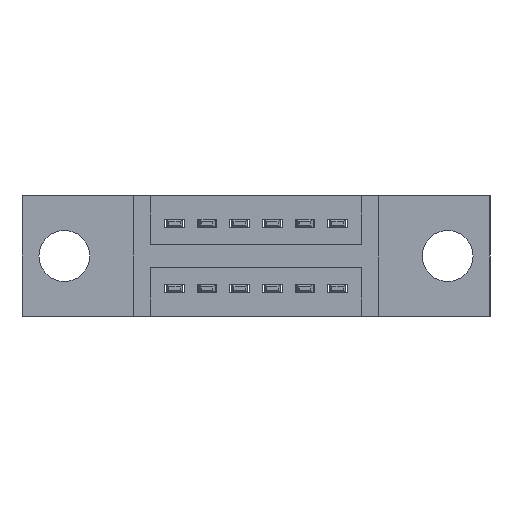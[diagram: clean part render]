
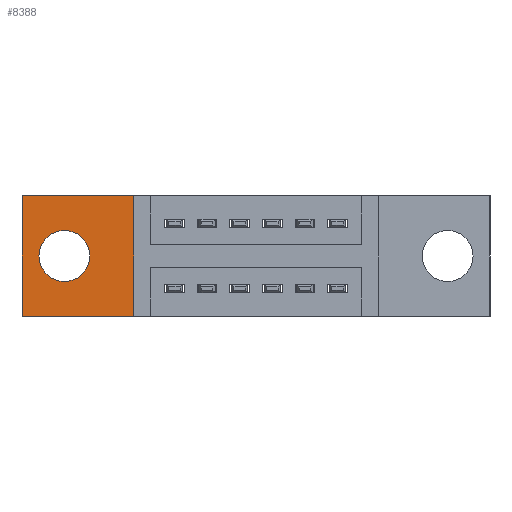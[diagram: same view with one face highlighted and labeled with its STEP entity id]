
A CAD part, front view. The second image highlights one B-rep face of the part: STEP entity #8388.
In plain terms, the highlighted planar face has unit normal (0, -1, 0).
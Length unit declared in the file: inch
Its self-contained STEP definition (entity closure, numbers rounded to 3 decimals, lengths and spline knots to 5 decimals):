
#304 = AXIS2_PLACEMENT_3D ( 'NONE', #477, #456, #7009 ) ;
#371 = AXIS2_PLACEMENT_3D ( 'NONE', #6355, #4152, #2954 ) ;
#456 = DIRECTION ( 'NONE',  ( 0., -1., 0. ) ) ;
#477 = CARTESIAN_POINT ( 'NONE',  ( 0., 0.17, -0.37 ) ) ;
#710 = VERTEX_POINT ( 'NONE', #9398 ) ;
#741 = EDGE_CURVE ( 'NONE', #1641, #5937, #3170, .T. ) ;
#893 = VECTOR ( 'NONE', #1954, 39.37008 ) ;
#1215 = CARTESIAN_POINT ( 'NONE',  ( 0.13, 0.17, -0.107 ) ) ;
#1598 = ORIENTED_EDGE ( 'NONE', *, *, #5074, .F. ) ;
#1641 = VERTEX_POINT ( 'NONE', #6620 ) ;
#1666 = CARTESIAN_POINT ( 'NONE',  ( 0., 0.17, 0. ) ) ;
#1954 = DIRECTION ( 'NONE',  ( 0., 0., -1. ) ) ;
#1985 = CARTESIAN_POINT ( 'NONE',  ( 0., 0.17, 0. ) ) ;
#2731 = PLANE ( 'NONE',  #304 ) ;
#2954 = DIRECTION ( 'NONE',  ( 0., 0., -1. ) ) ;
#3034 = CIRCLE ( 'NONE', #371, 0.078 ) ;
#3081 = ORIENTED_EDGE ( 'NONE', *, *, #9248, .F. ) ;
#3170 = LINE ( 'NONE', #1985, #893 ) ;
#3262 = AXIS2_PLACEMENT_3D ( 'NONE', #3743, #4475, #5957 ) ;
#3398 = VERTEX_POINT ( 'NONE', #1215 ) ;
#3563 = CARTESIAN_POINT ( 'NONE',  ( 0., 0.17, -0.37 ) ) ;
#3608 = VERTEX_POINT ( 'NONE', #4558 ) ;
#3743 = CARTESIAN_POINT ( 'NONE',  ( 0.13, 0.17, -0.185 ) ) ;
#3832 = DIRECTION ( 'NONE',  ( -1., 0., 0. ) ) ;
#3960 = VECTOR ( 'NONE', #3832, 39.37008 ) ;
#4073 = ORIENTED_EDGE ( 'NONE', *, *, #4602, .T. ) ;
#4152 = DIRECTION ( 'NONE',  ( 0., -1., 0. ) ) ;
#4201 = LINE ( 'NONE', #4662, #7805 ) ;
#4475 = DIRECTION ( 'NONE',  ( 0., -1., 0. ) ) ;
#4529 = ORIENTED_EDGE ( 'NONE', *, *, #741, .T. ) ;
#4558 = CARTESIAN_POINT ( 'NONE',  ( 0.13, 0.17, -0.263 ) ) ;
#4602 = EDGE_CURVE ( 'NONE', #5937, #710, #6333, .T. ) ;
#4662 = CARTESIAN_POINT ( 'NONE',  ( 0.3425, 0.17, 0. ) ) ;
#4689 = ORIENTED_EDGE ( 'NONE', *, *, #7722, .T. ) ;
#4899 = CARTESIAN_POINT ( 'NONE',  ( 0.3425, 0.17, 0. ) ) ;
#5042 = EDGE_LOOP ( 'NONE', ( #1598, #3081 ) ) ;
#5074 = EDGE_CURVE ( 'NONE', #3398, #3608, #6286, .T. ) ;
#5295 = EDGE_CURVE ( 'NONE', #8436, #1641, #9396, .T. ) ;
#5647 = EDGE_LOOP ( 'NONE', ( #4529, #4073, #4689, #7973 ) ) ;
#5930 = VECTOR ( 'NONE', #6534, 39.37008 ) ;
#5937 = VERTEX_POINT ( 'NONE', #3563 ) ;
#5957 = DIRECTION ( 'NONE',  ( 0., 0., -1. ) ) ;
#6045 = CARTESIAN_POINT ( 'NONE',  ( 0., 0.17, -0.37 ) ) ;
#6090 = DIRECTION ( 'NONE',  ( 0., 0., 1. ) ) ;
#6286 = CIRCLE ( 'NONE', #3262, 0.078 ) ;
#6333 = LINE ( 'NONE', #6045, #5930 ) ;
#6355 = CARTESIAN_POINT ( 'NONE',  ( 0.13, 0.17, -0.185 ) ) ;
#6378 = FACE_BOUND ( 'NONE', #5042, .T. ) ;
#6534 = DIRECTION ( 'NONE',  ( 1., 0., 0. ) ) ;
#6620 = CARTESIAN_POINT ( 'NONE',  ( 0., 0.17, 0. ) ) ;
#7009 = DIRECTION ( 'NONE',  ( 0., 0., -1. ) ) ;
#7550 = FACE_OUTER_BOUND ( 'NONE', #5647, .T. ) ;
#7722 = EDGE_CURVE ( 'NONE', #710, #8436, #4201, .T. ) ;
#7805 = VECTOR ( 'NONE', #6090, 39.37008 ) ;
#7973 = ORIENTED_EDGE ( 'NONE', *, *, #5295, .T. ) ;
#8388 = ADVANCED_FACE ( 'NONE', ( #6378, #7550 ), #2731, .T. ) ;
#8436 = VERTEX_POINT ( 'NONE', #4899 ) ;
#9248 = EDGE_CURVE ( 'NONE', #3608, #3398, #3034, .T. ) ;
#9396 = LINE ( 'NONE', #1666, #3960 ) ;
#9398 = CARTESIAN_POINT ( 'NONE',  ( 0.3425, 0.17, -0.37 ) ) ;
